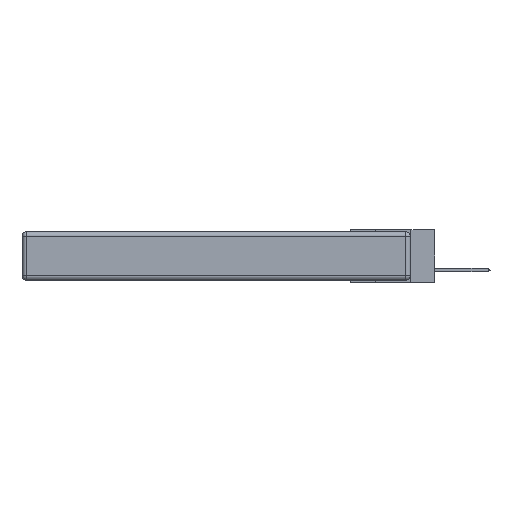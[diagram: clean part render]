
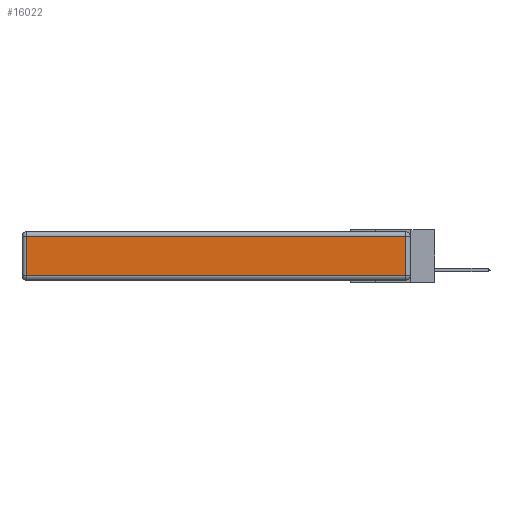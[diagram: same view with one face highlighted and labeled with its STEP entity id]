
A CAD part, left-side view. The second image highlights one B-rep face of the part: STEP entity #16022.
In plain terms, the highlighted planar face has unit normal (-1, 0, 0).
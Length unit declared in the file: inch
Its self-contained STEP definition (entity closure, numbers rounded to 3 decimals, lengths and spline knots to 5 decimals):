
#1804 = LINE ( 'NONE', #2901, #5688 ) ;
#2032 = PLANE ( 'NONE',  #16927 ) ;
#2053 = EDGE_CURVE ( 'NONE', #6468, #20165, #12788, .T. ) ;
#2901 = CARTESIAN_POINT ( 'NONE',  ( 0., 2.72, -0.343 ) ) ;
#3229 = FACE_OUTER_BOUND ( 'NONE', #17986, .T. ) ;
#3546 = ORIENTED_EDGE ( 'NONE', *, *, #8731, .T. ) ;
#5394 = CARTESIAN_POINT ( 'NONE',  ( 0., 0., -0.343 ) ) ;
#5462 = DIRECTION ( 'NONE',  ( 0., 0., 1. ) ) ;
#5688 = VECTOR ( 'NONE', #6649, 39.37008 ) ;
#6329 = CARTESIAN_POINT ( 'NONE',  ( 0., 0.03, -0.03 ) ) ;
#6468 = VERTEX_POINT ( 'NONE', #6329 ) ;
#6649 = DIRECTION ( 'NONE',  ( 0., 0., -1. ) ) ;
#7039 = CARTESIAN_POINT ( 'NONE',  ( 0., 2.72, -0.313 ) ) ;
#7117 = CARTESIAN_POINT ( 'NONE',  ( 0., 2.72, -0.03 ) ) ;
#8731 = EDGE_CURVE ( 'NONE', #20165, #20291, #1804, .T. ) ;
#8958 = CARTESIAN_POINT ( 'NONE',  ( 0., 0., -0.313 ) ) ;
#9233 = EDGE_CURVE ( 'NONE', #21140, #6468, #21835, .T. ) ;
#11011 = VECTOR ( 'NONE', #21352, 39.37008 ) ;
#12788 = LINE ( 'NONE', #22126, #22208 ) ;
#14372 = DIRECTION ( 'NONE',  ( -1., 0., 0. ) ) ;
#14538 = ORIENTED_EDGE ( 'NONE', *, *, #16561, .T. ) ;
#16022 = ADVANCED_FACE ( 'NONE', ( #3229 ), #2032, .T. ) ;
#16161 = ORIENTED_EDGE ( 'NONE', *, *, #2053, .T. ) ;
#16561 = EDGE_CURVE ( 'NONE', #20291, #21140, #18532, .T. ) ;
#16927 = AXIS2_PLACEMENT_3D ( 'NONE', #5394, #14372, #5462 ) ;
#17986 = EDGE_LOOP ( 'NONE', ( #14538, #18385, #16161, #3546 ) ) ;
#18385 = ORIENTED_EDGE ( 'NONE', *, *, #9233, .T. ) ;
#18408 = DIRECTION ( 'NONE',  ( 0., 1., 0. ) ) ;
#18532 = LINE ( 'NONE', #8958, #11011 ) ;
#18714 = CARTESIAN_POINT ( 'NONE',  ( 0., 0.03, -0.343 ) ) ;
#19070 = VECTOR ( 'NONE', #22369, 39.37008 ) ;
#19173 = CARTESIAN_POINT ( 'NONE',  ( 0., 0.03, -0.313 ) ) ;
#20165 = VERTEX_POINT ( 'NONE', #7117 ) ;
#20291 = VERTEX_POINT ( 'NONE', #7039 ) ;
#21140 = VERTEX_POINT ( 'NONE', #19173 ) ;
#21352 = DIRECTION ( 'NONE',  ( 0., -1., 0. ) ) ;
#21835 = LINE ( 'NONE', #18714, #19070 ) ;
#22126 = CARTESIAN_POINT ( 'NONE',  ( 0., 2.75, -0.03 ) ) ;
#22208 = VECTOR ( 'NONE', #18408, 39.37008 ) ;
#22369 = DIRECTION ( 'NONE',  ( 0., 0., 1. ) ) ;
